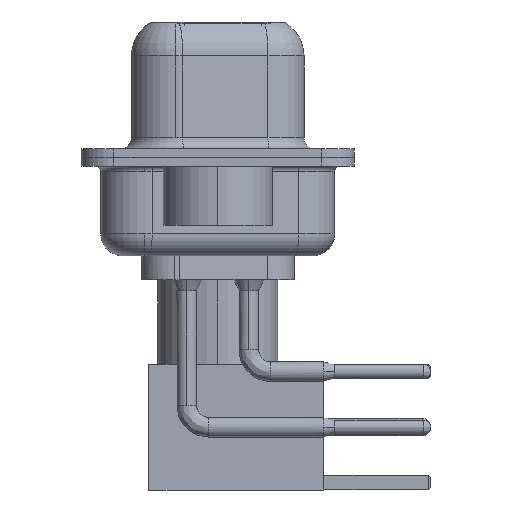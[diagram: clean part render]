
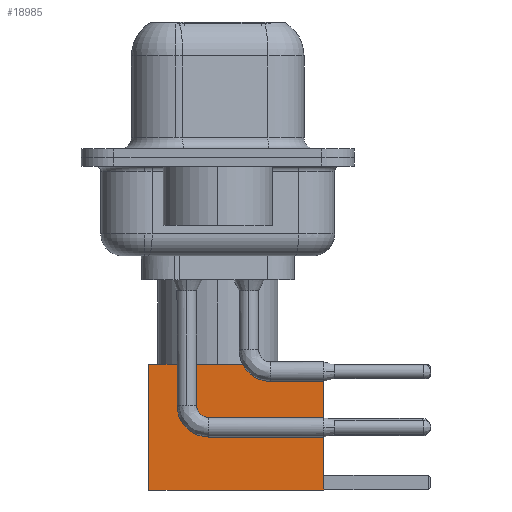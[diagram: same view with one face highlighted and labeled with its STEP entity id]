
A CAD part, left-side view. The second image highlights one B-rep face of the part: STEP entity #18985.
In plain terms, the highlighted face is planar.
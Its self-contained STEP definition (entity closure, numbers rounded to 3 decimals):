
#322 = DIRECTION ( 'NONE',  ( 0., 1., 0. ) ) ;
#1226 = CARTESIAN_POINT ( 'NONE',  ( -2.875, 2.875, 0. ) ) ;
#1751 = CARTESIAN_POINT ( 'NONE',  ( -2.875, 2.875, 8. ) ) ;
#2018 = ORIENTED_EDGE ( 'NONE', *, *, #17509, .F. ) ;
#2411 = VECTOR ( 'NONE', #13023, 1000. ) ;
#2632 = CARTESIAN_POINT ( 'NONE',  ( 2.875, 2.875, 0. ) ) ;
#2656 = CARTESIAN_POINT ( 'NONE',  ( -2.875, 2.875, 0. ) ) ;
#3214 = CARTESIAN_POINT ( 'NONE',  ( 0., 2.875, 8. ) ) ;
#3265 = VERTEX_POINT ( 'NONE', #13222 ) ;
#4338 = VERTEX_POINT ( 'NONE', #2656 ) ;
#6147 = LINE ( 'NONE', #3214, #2411 ) ;
#7060 = PLANE ( 'NONE',  #8994 ) ;
#7492 = EDGE_CURVE ( 'NONE', #10581, #4338, #18148, .T. ) ;
#8994 = AXIS2_PLACEMENT_3D ( 'NONE', #15593, #322, #15482 ) ;
#9277 = DIRECTION ( 'NONE',  ( 0., 0., -1. ) ) ;
#10558 = ORIENTED_EDGE ( 'NONE', *, *, #19165, .T. ) ;
#10581 = VERTEX_POINT ( 'NONE', #2632 ) ;
#10937 = LINE ( 'NONE', #17677, #16067 ) ;
#11663 = EDGE_CURVE ( 'NONE', #3265, #20875, #6147, .T. ) ;
#11852 = ORIENTED_EDGE ( 'NONE', *, *, #11663, .F. ) ;
#12390 = VECTOR ( 'NONE', #15073, 1000. ) ;
#12418 = EDGE_LOOP ( 'NONE', ( #10558, #16172, #2018, #11852 ) ) ;
#13023 = DIRECTION ( 'NONE',  ( -1., 0., 0. ) ) ;
#13026 = DIRECTION ( 'NONE',  ( 0., 0., -1. ) ) ;
#13222 = CARTESIAN_POINT ( 'NONE',  ( 2.875, 2.875, 8. ) ) ;
#14837 = CARTESIAN_POINT ( 'NONE',  ( 0., 2.875, 0. ) ) ;
#14931 = LINE ( 'NONE', #1226, #15309 ) ;
#15073 = DIRECTION ( 'NONE',  ( -1., 0., 0. ) ) ;
#15309 = VECTOR ( 'NONE', #13026, 1000. ) ;
#15482 = DIRECTION ( 'NONE',  ( 0., 0., 1. ) ) ;
#15593 = CARTESIAN_POINT ( 'NONE',  ( 2.875, 2.875, 0. ) ) ;
#16067 = VECTOR ( 'NONE', #9277, 1000. ) ;
#16172 = ORIENTED_EDGE ( 'NONE', *, *, #7492, .T. ) ;
#17509 = EDGE_CURVE ( 'NONE', #20875, #4338, #14931, .T. ) ;
#17677 = CARTESIAN_POINT ( 'NONE',  ( 2.875, 2.875, 0. ) ) ;
#18148 = LINE ( 'NONE', #14837, #12390 ) ;
#18985 = ADVANCED_FACE ( 'NONE', ( #20787 ), #7060, .T. ) ;
#19165 = EDGE_CURVE ( 'NONE', #3265, #10581, #10937, .T. ) ;
#20787 = FACE_OUTER_BOUND ( 'NONE', #12418, .T. ) ;
#20875 = VERTEX_POINT ( 'NONE', #1751 ) ;
